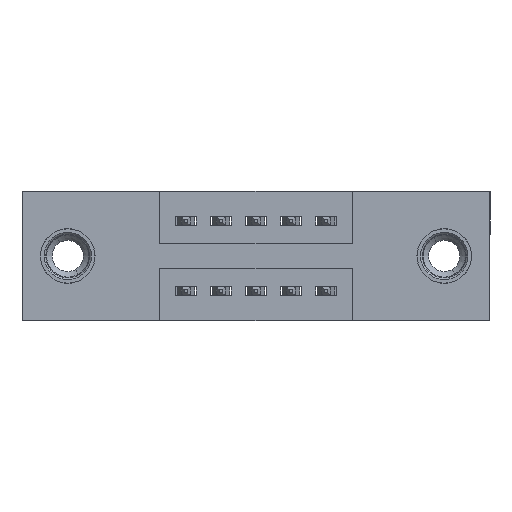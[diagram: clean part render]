
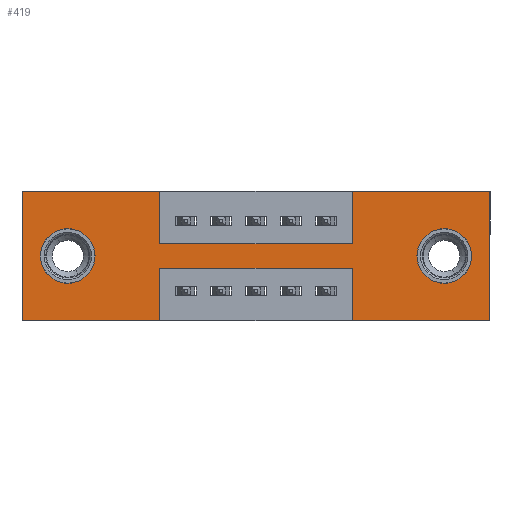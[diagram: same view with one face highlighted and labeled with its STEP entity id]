
A CAD part, front view. The second image highlights one B-rep face of the part: STEP entity #419.
In plain terms, the highlighted planar face has unit normal (0, -1, 0).
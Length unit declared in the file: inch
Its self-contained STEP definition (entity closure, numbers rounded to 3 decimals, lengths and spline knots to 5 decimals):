
#81 = CARTESIAN_POINT ( 'NONE',  ( 0.13, 0., -0.185 ) ) ;
#201 = CARTESIAN_POINT ( 'NONE',  ( 0., 0., -0.37 ) ) ;
#209 = EDGE_CURVE ( 'NONE', #4933, #12306, #10334, .T. ) ;
#280 = LINE ( 'NONE', #12840, #662 ) ;
#419 = ADVANCED_FACE ( 'NONE', ( #3247, #532, #11103 ), #13580, .T. ) ;
#447 = DIRECTION ( 'NONE',  ( -1., 0., 0. ) ) ;
#466 = DIRECTION ( 'NONE',  ( 1., 0., 0. ) ) ;
#532 = FACE_BOUND ( 'NONE', #4975, .T. ) ;
#662 = VECTOR ( 'NONE', #466, 39.37008 ) ;
#798 = DIRECTION ( 'NONE',  ( 0., 0., -1. ) ) ;
#946 = ORIENTED_EDGE ( 'NONE', *, *, #11461, .F. ) ;
#960 = VERTEX_POINT ( 'NONE', #4581 ) ;
#1029 = DIRECTION ( 'NONE',  ( 0., 1., 0. ) ) ;
#1044 = VERTEX_POINT ( 'NONE', #9005 ) ;
#1175 = ORIENTED_EDGE ( 'NONE', *, *, #12244, .F. ) ;
#1182 = CIRCLE ( 'NONE', #13074, 0.078 ) ;
#1203 = CARTESIAN_POINT ( 'NONE',  ( 0.9425, 0., -0.37 ) ) ;
#1286 = DIRECTION ( 'NONE',  ( 0., 0., 1. ) ) ;
#1389 = VECTOR ( 'NONE', #9430, 39.37008 ) ;
#1650 = ORIENTED_EDGE ( 'NONE', *, *, #11658, .T. ) ;
#2167 = CARTESIAN_POINT ( 'NONE',  ( 0.3925, 0., -0.37 ) ) ;
#2359 = DIRECTION ( 'NONE',  ( 1., 0., 0. ) ) ;
#2506 = CIRCLE ( 'NONE', #7083, 0.078 ) ;
#2569 = CARTESIAN_POINT ( 'NONE',  ( 0., 0., -0.37 ) ) ;
#2693 = CARTESIAN_POINT ( 'NONE',  ( 0., 0., 0. ) ) ;
#2823 = ORIENTED_EDGE ( 'NONE', *, *, #5781, .F. ) ;
#2858 = VERTEX_POINT ( 'NONE', #9529 ) ;
#2913 = EDGE_LOOP ( 'NONE', ( #12252, #1650 ) ) ;
#2958 = EDGE_CURVE ( 'NONE', #8827, #3852, #280, .T. ) ;
#3043 = AXIS2_PLACEMENT_3D ( 'NONE', #81, #7742, #1286 ) ;
#3137 = CARTESIAN_POINT ( 'NONE',  ( 0.9425, 0., 0. ) ) ;
#3247 = FACE_BOUND ( 'NONE', #2913, .T. ) ;
#3465 = CARTESIAN_POINT ( 'NONE',  ( 0., 0., -0.37 ) ) ;
#3487 = ORIENTED_EDGE ( 'NONE', *, *, #9873, .T. ) ;
#3600 = EDGE_LOOP ( 'NONE', ( #10126, #946, #7272, #2823, #7111, #12802, #13142, #5178, #10286, #11606, #1175, #9064 ) ) ;
#3631 = CARTESIAN_POINT ( 'NONE',  ( 0.3925, 0., -0.15 ) ) ;
#3665 = DIRECTION ( 'NONE',  ( -1., 0., 0. ) ) ;
#3722 = VERTEX_POINT ( 'NONE', #3137 ) ;
#3776 = EDGE_CURVE ( 'NONE', #3852, #3722, #7770, .T. ) ;
#3852 = VERTEX_POINT ( 'NONE', #13329 ) ;
#3868 = CARTESIAN_POINT ( 'NONE',  ( 0.3925, 0., -0.22 ) ) ;
#3927 = CARTESIAN_POINT ( 'NONE',  ( 1.205, 0., -0.185 ) ) ;
#4094 = LINE ( 'NONE', #201, #9199 ) ;
#4177 = EDGE_CURVE ( 'NONE', #5900, #9984, #10185, .T. ) ;
#4344 = AXIS2_PLACEMENT_3D ( 'NONE', #3465, #13196, #13248 ) ;
#4581 = CARTESIAN_POINT ( 'NONE',  ( 0.13, 0., -0.263 ) ) ;
#4746 = DIRECTION ( 'NONE',  ( -1., 0., 0. ) ) ;
#4782 = DIRECTION ( 'NONE',  ( 0., 0., 1. ) ) ;
#4924 = CIRCLE ( 'NONE', #3043, 0.078 ) ;
#4933 = VERTEX_POINT ( 'NONE', #7287 ) ;
#4975 = EDGE_LOOP ( 'NONE', ( #7363, #3487 ) ) ;
#5005 = DIRECTION ( 'NONE',  ( 0., 0., -1. ) ) ;
#5039 = VECTOR ( 'NONE', #4782, 39.37008 ) ;
#5178 = ORIENTED_EDGE ( 'NONE', *, *, #2958, .F. ) ;
#5259 = DIRECTION ( 'NONE',  ( 0., 1., 0. ) ) ;
#5638 = VERTEX_POINT ( 'NONE', #13490 ) ;
#5781 = EDGE_CURVE ( 'NONE', #9726, #10700, #4094, .T. ) ;
#5814 = CIRCLE ( 'NONE', #7916, 0.078 ) ;
#5900 = VERTEX_POINT ( 'NONE', #5957 ) ;
#5957 = CARTESIAN_POINT ( 'NONE',  ( 0.3925, 0., -0.22 ) ) ;
#6244 = CARTESIAN_POINT ( 'NONE',  ( 0.3925, 0., 0. ) ) ;
#6279 = VECTOR ( 'NONE', #798, 39.37008 ) ;
#6358 = EDGE_CURVE ( 'NONE', #11570, #960, #4924, .T. ) ;
#6683 = EDGE_CURVE ( 'NONE', #10700, #7013, #9814, .T. ) ;
#7013 = VERTEX_POINT ( 'NONE', #12816 ) ;
#7083 = AXIS2_PLACEMENT_3D ( 'NONE', #7508, #1029, #8524 ) ;
#7111 = ORIENTED_EDGE ( 'NONE', *, *, #9548, .F. ) ;
#7149 = LINE ( 'NONE', #8457, #1389 ) ;
#7164 = CARTESIAN_POINT ( 'NONE',  ( 0.9425, 0., -0.37 ) ) ;
#7192 = DIRECTION ( 'NONE',  ( 1., 0., 0. ) ) ;
#7272 = ORIENTED_EDGE ( 'NONE', *, *, #6683, .F. ) ;
#7287 = CARTESIAN_POINT ( 'NONE',  ( 0., 0., 0. ) ) ;
#7363 = ORIENTED_EDGE ( 'NONE', *, *, #6358, .T. ) ;
#7486 = CARTESIAN_POINT ( 'NONE',  ( 0.3925, 0., 0. ) ) ;
#7508 = CARTESIAN_POINT ( 'NONE',  ( 1.205, 0., -0.185 ) ) ;
#7539 = VECTOR ( 'NONE', #13252, 39.37008 ) ;
#7688 = VECTOR ( 'NONE', #2359, 39.37008 ) ;
#7742 = DIRECTION ( 'NONE',  ( 0., 1., 0. ) ) ;
#7770 = LINE ( 'NONE', #12629, #5039 ) ;
#7916 = AXIS2_PLACEMENT_3D ( 'NONE', #11303, #5259, #12334 ) ;
#8043 = EDGE_CURVE ( 'NONE', #3722, #5638, #12461, .T. ) ;
#8168 = DIRECTION ( 'NONE',  ( 0., 0., 1. ) ) ;
#8189 = VECTOR ( 'NONE', #8664, 39.37008 ) ;
#8457 = CARTESIAN_POINT ( 'NONE',  ( 0., 0., 0. ) ) ;
#8524 = DIRECTION ( 'NONE',  ( 0., 0., -1. ) ) ;
#8664 = DIRECTION ( 'NONE',  ( 0., 0., -1. ) ) ;
#8827 = VERTEX_POINT ( 'NONE', #3631 ) ;
#9005 = CARTESIAN_POINT ( 'NONE',  ( 0., 0., -0.37 ) ) ;
#9064 = ORIENTED_EDGE ( 'NONE', *, *, #11883, .F. ) ;
#9199 = VECTOR ( 'NONE', #4746, 39.37008 ) ;
#9430 = DIRECTION ( 'NONE',  ( 0., 0., 1. ) ) ;
#9529 = CARTESIAN_POINT ( 'NONE',  ( 1.205, 0., -0.107 ) ) ;
#9548 = EDGE_CURVE ( 'NONE', #5638, #9726, #10838, .T. ) ;
#9726 = VERTEX_POINT ( 'NONE', #11898 ) ;
#9814 = LINE ( 'NONE', #7164, #12186 ) ;
#9873 = EDGE_CURVE ( 'NONE', #960, #11570, #5814, .T. ) ;
#9958 = VECTOR ( 'NONE', #447, 39.37008 ) ;
#9984 = VERTEX_POINT ( 'NONE', #2167 ) ;
#10081 = VECTOR ( 'NONE', #7192, 39.37008 ) ;
#10126 = ORIENTED_EDGE ( 'NONE', *, *, #4177, .F. ) ;
#10185 = LINE ( 'NONE', #10377, #7539 ) ;
#10286 = ORIENTED_EDGE ( 'NONE', *, *, #10457, .F. ) ;
#10334 = LINE ( 'NONE', #2693, #7688 ) ;
#10377 = CARTESIAN_POINT ( 'NONE',  ( 0.3925, 0., -0.37 ) ) ;
#10457 = EDGE_CURVE ( 'NONE', #12306, #8827, #12266, .T. ) ;
#10493 = CARTESIAN_POINT ( 'NONE',  ( 1.335, 0., 0. ) ) ;
#10700 = VERTEX_POINT ( 'NONE', #1203 ) ;
#10838 = LINE ( 'NONE', #10493, #8189 ) ;
#11050 = DIRECTION ( 'NONE',  ( 0., 1., 0. ) ) ;
#11103 = FACE_OUTER_BOUND ( 'NONE', #3600, .T. ) ;
#11194 = VECTOR ( 'NONE', #3665, 39.37008 ) ;
#11303 = CARTESIAN_POINT ( 'NONE',  ( 0.13, 0., -0.185 ) ) ;
#11461 = EDGE_CURVE ( 'NONE', #7013, #5900, #12652, .T. ) ;
#11570 = VERTEX_POINT ( 'NONE', #12202 ) ;
#11606 = ORIENTED_EDGE ( 'NONE', *, *, #209, .F. ) ;
#11658 = EDGE_CURVE ( 'NONE', #12134, #2858, #2506, .T. ) ;
#11883 = EDGE_CURVE ( 'NONE', #9984, #1044, #13625, .T. ) ;
#11898 = CARTESIAN_POINT ( 'NONE',  ( 1.335, 0., -0.37 ) ) ;
#12134 = VERTEX_POINT ( 'NONE', #13280 ) ;
#12186 = VECTOR ( 'NONE', #8168, 39.37008 ) ;
#12202 = CARTESIAN_POINT ( 'NONE',  ( 0.13, 0., -0.107 ) ) ;
#12244 = EDGE_CURVE ( 'NONE', #1044, #4933, #7149, .T. ) ;
#12252 = ORIENTED_EDGE ( 'NONE', *, *, #12505, .T. ) ;
#12266 = LINE ( 'NONE', #6244, #6279 ) ;
#12306 = VERTEX_POINT ( 'NONE', #7486 ) ;
#12334 = DIRECTION ( 'NONE',  ( 0., 0., 1. ) ) ;
#12461 = LINE ( 'NONE', #13237, #10081 ) ;
#12505 = EDGE_CURVE ( 'NONE', #2858, #12134, #1182, .T. ) ;
#12629 = CARTESIAN_POINT ( 'NONE',  ( 0.9425, 0., 0. ) ) ;
#12652 = LINE ( 'NONE', #3868, #9958 ) ;
#12802 = ORIENTED_EDGE ( 'NONE', *, *, #8043, .F. ) ;
#12816 = CARTESIAN_POINT ( 'NONE',  ( 0.9425, 0., -0.22 ) ) ;
#12840 = CARTESIAN_POINT ( 'NONE',  ( 0.3925, 0., -0.15 ) ) ;
#13074 = AXIS2_PLACEMENT_3D ( 'NONE', #3927, #11050, #5005 ) ;
#13142 = ORIENTED_EDGE ( 'NONE', *, *, #3776, .F. ) ;
#13196 = DIRECTION ( 'NONE',  ( 0., -1., 0. ) ) ;
#13237 = CARTESIAN_POINT ( 'NONE',  ( 0., 0., 0. ) ) ;
#13248 = DIRECTION ( 'NONE',  ( 0., 0., -1. ) ) ;
#13252 = DIRECTION ( 'NONE',  ( 0., 0., -1. ) ) ;
#13280 = CARTESIAN_POINT ( 'NONE',  ( 1.205, 0., -0.263 ) ) ;
#13329 = CARTESIAN_POINT ( 'NONE',  ( 0.9425, 0., -0.15 ) ) ;
#13490 = CARTESIAN_POINT ( 'NONE',  ( 1.335, 0., 0. ) ) ;
#13580 = PLANE ( 'NONE',  #4344 ) ;
#13625 = LINE ( 'NONE', #2569, #11194 ) ;
